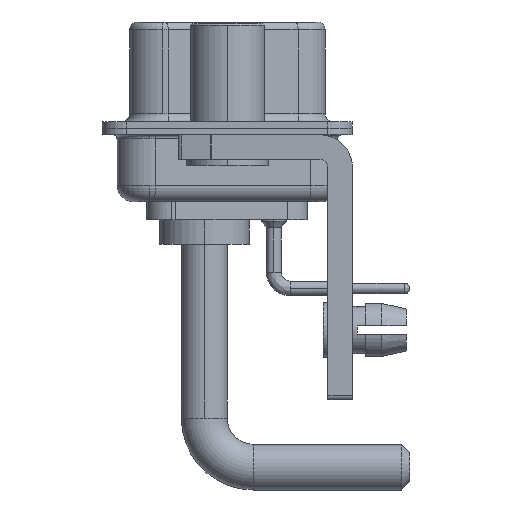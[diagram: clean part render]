
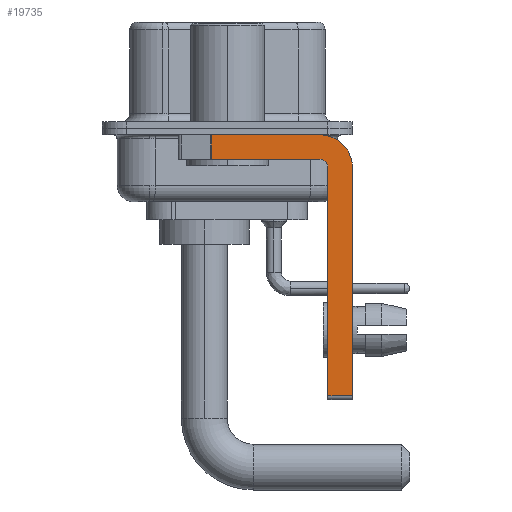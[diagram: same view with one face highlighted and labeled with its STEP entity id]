
A CAD part, left-side view. The second image highlights one B-rep face of the part: STEP entity #19735.
In plain terms, the highlighted planar face has unit normal (-1, 0, 0).
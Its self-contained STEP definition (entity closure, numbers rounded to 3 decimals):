
#443 = CARTESIAN_POINT ( 'NONE',  ( -2.9, -6.15, -16.6 ) ) ;
#610 = AXIS2_PLACEMENT_3D ( 'NONE', #21667, #6859, #8656 ) ;
#1110 = VECTOR ( 'NONE', #4516, 1000. ) ;
#1428 = EDGE_CURVE ( 'NONE', #22222, #16033, #19999, .T. ) ;
#1444 = CARTESIAN_POINT ( 'NONE',  ( -2.9, 0.978, -0.4 ) ) ;
#1591 = CARTESIAN_POINT ( 'NONE',  ( -2.9, -5.65, -16.35 ) ) ;
#1603 = LINE ( 'NONE', #24910, #9270 ) ;
#1678 = DIRECTION ( 'NONE',  ( 0., 0., -1. ) ) ;
#1761 = EDGE_CURVE ( 'NONE', #4294, #22399, #12641, .T. ) ;
#2264 = VECTOR ( 'NONE', #23479, 1000. ) ;
#2470 = DIRECTION ( 'NONE',  ( 0., 0., -1. ) ) ;
#2628 = EDGE_CURVE ( 'NONE', #9932, #4294, #6819, .T. ) ;
#2735 = FACE_OUTER_BOUND ( 'NONE', #21930, .T. ) ;
#2759 = AXIS2_PLACEMENT_3D ( 'NONE', #13210, #11403, #21531 ) ;
#3341 = VERTEX_POINT ( 'NONE', #11964 ) ;
#3673 = ORIENTED_EDGE ( 'NONE', *, *, #7168, .F. ) ;
#4145 = ORIENTED_EDGE ( 'NONE', *, *, #1428, .F. ) ;
#4294 = VERTEX_POINT ( 'NONE', #26749 ) ;
#4516 = DIRECTION ( 'NONE',  ( 0., 0., -1. ) ) ;
#5082 = CARTESIAN_POINT ( 'NONE',  ( -2.9, -5.65, -2.4 ) ) ;
#5126 = VERTEX_POINT ( 'NONE', #19802 ) ;
#6819 = CIRCLE ( 'NONE', #610, 2. ) ;
#6859 = DIRECTION ( 'NONE',  ( 1., 0., 0. ) ) ;
#7168 = EDGE_CURVE ( 'NONE', #5126, #22222, #19170, .T. ) ;
#7296 = AXIS2_PLACEMENT_3D ( 'NONE', #5082, #13542, #2470 ) ;
#7489 = DIRECTION ( 'NONE',  ( 0., 1., 0. ) ) ;
#8656 = DIRECTION ( 'NONE',  ( 0., 0., -1. ) ) ;
#9270 = VECTOR ( 'NONE', #9933, 1000. ) ;
#9644 = CARTESIAN_POINT ( 'NONE',  ( -2.9, -6.15, -2.4 ) ) ;
#9932 = VERTEX_POINT ( 'NONE', #17712 ) ;
#9933 = DIRECTION ( 'NONE',  ( 0., -1., 0. ) ) ;
#11183 = PLANE ( 'NONE',  #7296 ) ;
#11403 = DIRECTION ( 'NONE',  ( -1., 0., 0. ) ) ;
#11964 = CARTESIAN_POINT ( 'NONE',  ( -2.9, 0.978, -1.9 ) ) ;
#12641 = LINE ( 'NONE', #20674, #16462 ) ;
#13210 = CARTESIAN_POINT ( 'NONE',  ( -2.9, -5.65, -2.4 ) ) ;
#13232 = CARTESIAN_POINT ( 'NONE',  ( -2.9, 0.978, -1.9 ) ) ;
#13542 = DIRECTION ( 'NONE',  ( 1., 0., 0. ) ) ;
#16033 = VERTEX_POINT ( 'NONE', #23283 ) ;
#16462 = VECTOR ( 'NONE', #1678, 1000. ) ;
#16715 = ORIENTED_EDGE ( 'NONE', *, *, #24685, .F. ) ;
#17712 = CARTESIAN_POINT ( 'NONE',  ( -2.9, -5.65, -0.4 ) ) ;
#18180 = VECTOR ( 'NONE', #7489, 1000. ) ;
#18274 = EDGE_CURVE ( 'NONE', #5126, #22399, #27119, .T. ) ;
#19124 = ORIENTED_EDGE ( 'NONE', *, *, #2628, .F. ) ;
#19170 = LINE ( 'NONE', #443, #2264 ) ;
#19735 = ADVANCED_FACE ( 'NONE', ( #2735 ), #11183, .F. ) ;
#19802 = CARTESIAN_POINT ( 'NONE',  ( -2.9, -6.15, -16.35 ) ) ;
#19952 = CARTESIAN_POINT ( 'NONE',  ( -2.9, -5.65, -1.9 ) ) ;
#19999 = CIRCLE ( 'NONE', #2759, 0.5 ) ;
#20093 = LINE ( 'NONE', #19952, #18180 ) ;
#20175 = EDGE_CURVE ( 'NONE', #26771, #3341, #25877, .T. ) ;
#20674 = CARTESIAN_POINT ( 'NONE',  ( -2.9, -7.65, -2.4 ) ) ;
#20722 = CARTESIAN_POINT ( 'NONE',  ( -2.9, -7.65, -16.35 ) ) ;
#21531 = DIRECTION ( 'NONE',  ( 0., 0., 1. ) ) ;
#21667 = CARTESIAN_POINT ( 'NONE',  ( -2.9, -5.65, -2.4 ) ) ;
#21930 = EDGE_LOOP ( 'NONE', ( #16715, #23387, #24887, #4145, #3673, #24479, #26974, #19124 ) ) ;
#22222 = VERTEX_POINT ( 'NONE', #9644 ) ;
#22399 = VERTEX_POINT ( 'NONE', #20722 ) ;
#23283 = CARTESIAN_POINT ( 'NONE',  ( -2.9, -5.65, -1.9 ) ) ;
#23387 = ORIENTED_EDGE ( 'NONE', *, *, #20175, .T. ) ;
#23479 = DIRECTION ( 'NONE',  ( 0., 0., 1. ) ) ;
#24479 = ORIENTED_EDGE ( 'NONE', *, *, #18274, .T. ) ;
#24685 = EDGE_CURVE ( 'NONE', #26771, #9932, #1603, .T. ) ;
#24887 = ORIENTED_EDGE ( 'NONE', *, *, #25682, .F. ) ;
#24910 = CARTESIAN_POINT ( 'NONE',  ( -2.9, 3., -0.4 ) ) ;
#25032 = DIRECTION ( 'NONE',  ( 0., -1., 0. ) ) ;
#25387 = VECTOR ( 'NONE', #25032, 1000. ) ;
#25682 = EDGE_CURVE ( 'NONE', #16033, #3341, #20093, .T. ) ;
#25877 = LINE ( 'NONE', #13232, #1110 ) ;
#26749 = CARTESIAN_POINT ( 'NONE',  ( -2.9, -7.65, -2.4 ) ) ;
#26771 = VERTEX_POINT ( 'NONE', #1444 ) ;
#26974 = ORIENTED_EDGE ( 'NONE', *, *, #1761, .F. ) ;
#27119 = LINE ( 'NONE', #1591, #25387 ) ;
